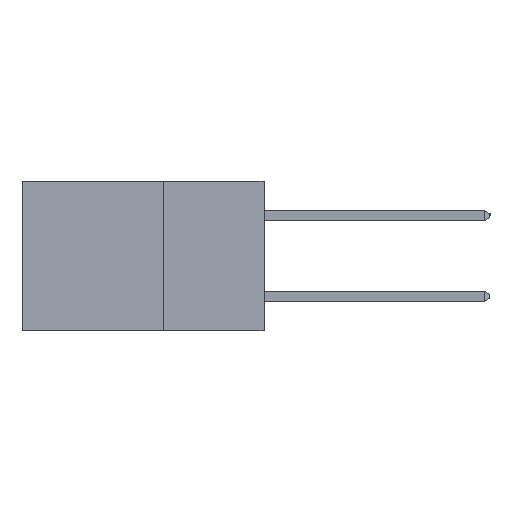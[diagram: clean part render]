
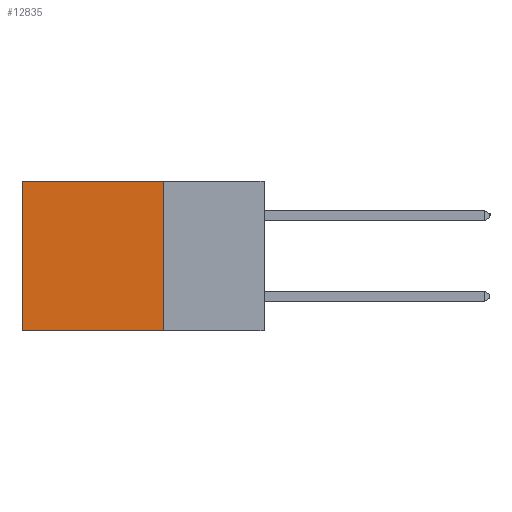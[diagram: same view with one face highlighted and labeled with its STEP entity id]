
A CAD part, left-side view. The second image highlights one B-rep face of the part: STEP entity #12835.
In plain terms, the highlighted planar face has unit normal (-1, 0, 0).
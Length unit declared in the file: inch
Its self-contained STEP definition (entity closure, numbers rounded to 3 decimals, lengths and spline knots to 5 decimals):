
#298 = VECTOR ( 'NONE', #11653, 39.37008 ) ;
#654 = CARTESIAN_POINT ( 'NONE',  ( 0.2615, 0.25, -0.37 ) ) ;
#2986 = EDGE_LOOP ( 'NONE', ( #16299, #15307, #5423, #10889 ) ) ;
#3062 = EDGE_CURVE ( 'NONE', #18189, #7543, #11208, .T. ) ;
#3139 = DIRECTION ( 'NONE',  ( 0., 1., 0. ) ) ;
#3314 = VERTEX_POINT ( 'NONE', #3956 ) ;
#3438 = DIRECTION ( 'NONE',  ( 0., 0., -1. ) ) ;
#3916 = EDGE_CURVE ( 'NONE', #8271, #18189, #4616, .T. ) ;
#3956 = CARTESIAN_POINT ( 'NONE',  ( 0.2615, 0.25, -0.37 ) ) ;
#4152 = PLANE ( 'NONE',  #15928 ) ;
#4409 = VECTOR ( 'NONE', #8097, 39.37008 ) ;
#4465 = EDGE_CURVE ( 'NONE', #8271, #3314, #12407, .T. ) ;
#4616 = LINE ( 'NONE', #10575, #9950 ) ;
#5147 = DIRECTION ( 'NONE',  ( 0., 0., -1. ) ) ;
#5423 = ORIENTED_EDGE ( 'NONE', *, *, #4465, .F. ) ;
#7044 = CARTESIAN_POINT ( 'NONE',  ( 0.2615, 0.6, 0. ) ) ;
#7543 = VERTEX_POINT ( 'NONE', #13274 ) ;
#8097 = DIRECTION ( 'NONE',  ( 0., 0., -1. ) ) ;
#8271 = VERTEX_POINT ( 'NONE', #18282 ) ;
#9950 = VECTOR ( 'NONE', #3139, 39.37008 ) ;
#10118 = CARTESIAN_POINT ( 'NONE',  ( 0.2615, 0.25, -0.37 ) ) ;
#10160 = CARTESIAN_POINT ( 'NONE',  ( 0.2615, 0.25, -0.37 ) ) ;
#10575 = CARTESIAN_POINT ( 'NONE',  ( 0.2615, 0.25, 0. ) ) ;
#10889 = ORIENTED_EDGE ( 'NONE', *, *, #3916, .T. ) ;
#11208 = LINE ( 'NONE', #14235, #17067 ) ;
#11653 = DIRECTION ( 'NONE',  ( 0., 1., 0. ) ) ;
#12407 = LINE ( 'NONE', #654, #4409 ) ;
#12835 = ADVANCED_FACE ( 'NONE', ( #17606 ), #4152, .F. ) ;
#13274 = CARTESIAN_POINT ( 'NONE',  ( 0.2615, 0.6, -0.37 ) ) ;
#13615 = EDGE_CURVE ( 'NONE', #3314, #7543, #19299, .T. ) ;
#14235 = CARTESIAN_POINT ( 'NONE',  ( 0.2615, 0.6, -0.37 ) ) ;
#15307 = ORIENTED_EDGE ( 'NONE', *, *, #13615, .F. ) ;
#15928 = AXIS2_PLACEMENT_3D ( 'NONE', #10118, #16123, #3438 ) ;
#16123 = DIRECTION ( 'NONE',  ( 1., 0., 0. ) ) ;
#16299 = ORIENTED_EDGE ( 'NONE', *, *, #3062, .T. ) ;
#17067 = VECTOR ( 'NONE', #5147, 39.37008 ) ;
#17606 = FACE_OUTER_BOUND ( 'NONE', #2986, .T. ) ;
#18189 = VERTEX_POINT ( 'NONE', #7044 ) ;
#18282 = CARTESIAN_POINT ( 'NONE',  ( 0.2615, 0.25, 0. ) ) ;
#19299 = LINE ( 'NONE', #10160, #298 ) ;
